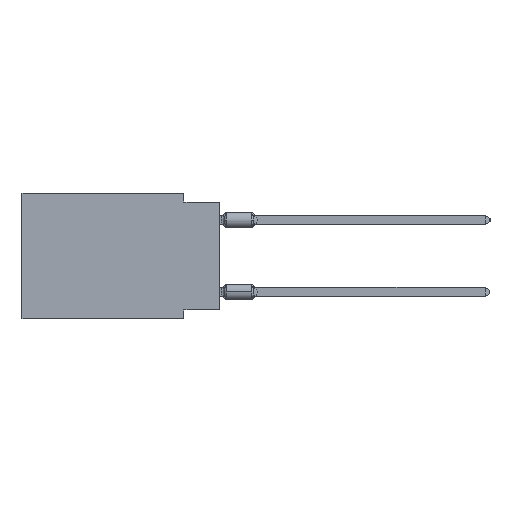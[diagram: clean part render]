
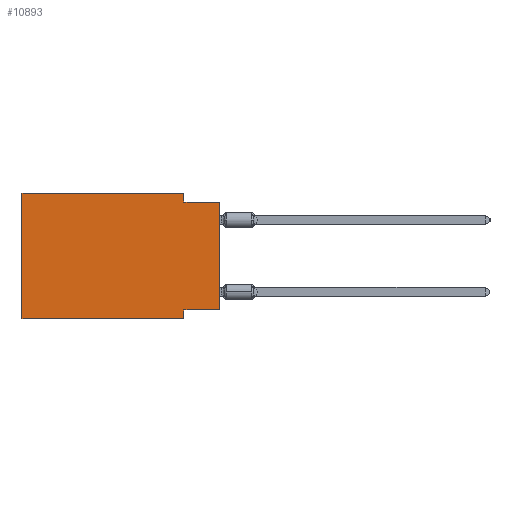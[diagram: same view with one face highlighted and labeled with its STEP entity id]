
A CAD part, left-side view. The second image highlights one B-rep face of the part: STEP entity #10893.
In plain terms, the highlighted planar face has unit normal (-1, 0, 0).
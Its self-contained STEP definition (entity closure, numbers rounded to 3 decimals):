
#206 = CARTESIAN_POINT ( 'NONE',  ( 0., 13.97, -8.89 ) ) ;
#1264 = LINE ( 'NONE', #17097, #17489 ) ;
#1799 = ORIENTED_EDGE ( 'NONE', *, *, #18202, .F. ) ;
#1887 = VERTEX_POINT ( 'NONE', #5600 ) ;
#2038 = CARTESIAN_POINT ( 'NONE',  ( 0., 0., 0. ) ) ;
#2090 = VECTOR ( 'NONE', #11003, 1000. ) ;
#2111 = VECTOR ( 'NONE', #2860, 1000. ) ;
#2294 = LINE ( 'NONE', #13145, #28364 ) ;
#2515 = PLANE ( 'NONE',  #14867 ) ;
#2860 = DIRECTION ( 'NONE',  ( 0., -1., 0. ) ) ;
#2996 = DIRECTION ( 'NONE',  ( 0., -1., 0. ) ) ;
#3589 = VECTOR ( 'NONE', #17853, 1000. ) ;
#3655 = VERTEX_POINT ( 'NONE', #11421 ) ;
#3973 = DIRECTION ( 'NONE',  ( 0., -1., 0. ) ) ;
#5059 = CARTESIAN_POINT ( 'NONE',  ( 0., 0., -0.635 ) ) ;
#5395 = ORIENTED_EDGE ( 'NONE', *, *, #12679, .F. ) ;
#5600 = CARTESIAN_POINT ( 'NONE',  ( 0., 13.97, 0. ) ) ;
#5760 = CARTESIAN_POINT ( 'NONE',  ( 0., 13.97, 0. ) ) ;
#5957 = DIRECTION ( 'NONE',  ( 0., 0., 1. ) ) ;
#6166 = LINE ( 'NONE', #15108, #20729 ) ;
#6353 = VERTEX_POINT ( 'NONE', #14256 ) ;
#6766 = DIRECTION ( 'NONE',  ( 0., 0., -1. ) ) ;
#7111 = LINE ( 'NONE', #5059, #2111 ) ;
#7874 = CARTESIAN_POINT ( 'NONE',  ( 0., 0., -0.635 ) ) ;
#8122 = EDGE_LOOP ( 'NONE', ( #23179, #5395, #21711, #1799, #10453, #18465, #12588, #13521 ) ) ;
#9933 = EDGE_CURVE ( 'NONE', #11052, #15423, #15659, .T. ) ;
#10393 = EDGE_CURVE ( 'NONE', #3655, #6353, #2294, .T. ) ;
#10453 = ORIENTED_EDGE ( 'NONE', *, *, #22115, .F. ) ;
#10893 = ADVANCED_FACE ( 'NONE', ( #16286 ), #2515, .F. ) ;
#10996 = CARTESIAN_POINT ( 'NONE',  ( 0., 0., -8.255 ) ) ;
#11003 = DIRECTION ( 'NONE',  ( 0., 0., 1. ) ) ;
#11052 = VERTEX_POINT ( 'NONE', #16435 ) ;
#11251 = DIRECTION ( 'NONE',  ( 0., 0., -1. ) ) ;
#11421 = CARTESIAN_POINT ( 'NONE',  ( 0., 2.54, 0. ) ) ;
#12224 = EDGE_CURVE ( 'NONE', #11052, #28190, #24292, .T. ) ;
#12588 = ORIENTED_EDGE ( 'NONE', *, *, #21287, .F. ) ;
#12679 = EDGE_CURVE ( 'NONE', #6353, #28190, #7111, .T. ) ;
#13145 = CARTESIAN_POINT ( 'NONE',  ( 0., 2.54, 0. ) ) ;
#13367 = DIRECTION ( 'NONE',  ( 1., 0., 0. ) ) ;
#13521 = ORIENTED_EDGE ( 'NONE', *, *, #9933, .F. ) ;
#14256 = CARTESIAN_POINT ( 'NONE',  ( 0., 2.54, -0.635 ) ) ;
#14867 = AXIS2_PLACEMENT_3D ( 'NONE', #18038, #13367, #6766 ) ;
#15108 = CARTESIAN_POINT ( 'NONE',  ( 0., 13.97, -8.89 ) ) ;
#15423 = VERTEX_POINT ( 'NONE', #24822 ) ;
#15425 = VERTEX_POINT ( 'NONE', #206 ) ;
#15659 = LINE ( 'NONE', #10996, #3589 ) ;
#16286 = FACE_OUTER_BOUND ( 'NONE', #8122, .T. ) ;
#16435 = CARTESIAN_POINT ( 'NONE',  ( 0., 0., -8.255 ) ) ;
#17097 = CARTESIAN_POINT ( 'NONE',  ( 0., 13.97, 0. ) ) ;
#17489 = VECTOR ( 'NONE', #5957, 1000. ) ;
#17593 = CARTESIAN_POINT ( 'NONE',  ( 0., 2.54, -8.89 ) ) ;
#17853 = DIRECTION ( 'NONE',  ( 0., 1., 0. ) ) ;
#18038 = CARTESIAN_POINT ( 'NONE',  ( 0., 13.97, 0. ) ) ;
#18202 = EDGE_CURVE ( 'NONE', #1887, #3655, #25664, .T. ) ;
#18465 = ORIENTED_EDGE ( 'NONE', *, *, #21405, .T. ) ;
#20233 = LINE ( 'NONE', #17593, #26772 ) ;
#20729 = VECTOR ( 'NONE', #3973, 1000. ) ;
#21287 = EDGE_CURVE ( 'NONE', #15423, #26123, #20233, .T. ) ;
#21405 = EDGE_CURVE ( 'NONE', #15425, #26123, #6166, .T. ) ;
#21711 = ORIENTED_EDGE ( 'NONE', *, *, #10393, .F. ) ;
#21983 = DIRECTION ( 'NONE',  ( 0., 0., -1. ) ) ;
#22115 = EDGE_CURVE ( 'NONE', #15425, #1887, #1264, .T. ) ;
#23179 = ORIENTED_EDGE ( 'NONE', *, *, #12224, .T. ) ;
#24292 = LINE ( 'NONE', #2038, #2090 ) ;
#24822 = CARTESIAN_POINT ( 'NONE',  ( 0., 2.54, -8.255 ) ) ;
#25664 = LINE ( 'NONE', #5760, #27445 ) ;
#26123 = VERTEX_POINT ( 'NONE', #27427 ) ;
#26772 = VECTOR ( 'NONE', #21983, 1000. ) ;
#27427 = CARTESIAN_POINT ( 'NONE',  ( 0., 2.54, -8.89 ) ) ;
#27445 = VECTOR ( 'NONE', #2996, 1000. ) ;
#28190 = VERTEX_POINT ( 'NONE', #7874 ) ;
#28364 = VECTOR ( 'NONE', #11251, 1000. ) ;
